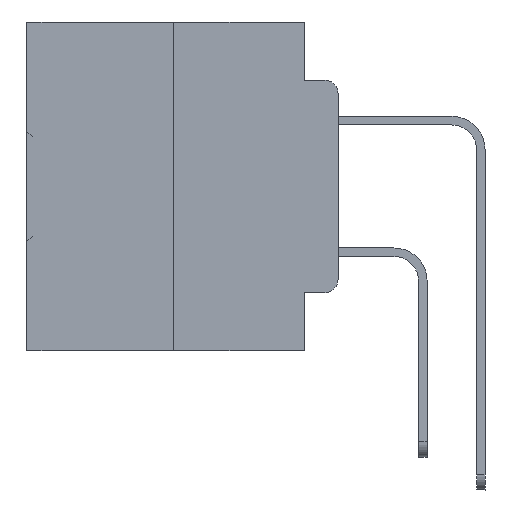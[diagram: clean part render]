
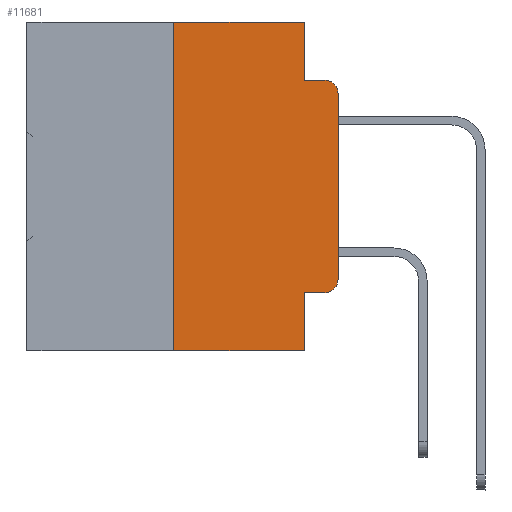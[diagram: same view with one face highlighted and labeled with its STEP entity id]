
A CAD part, left-side view. The second image highlights one B-rep face of the part: STEP entity #11681.
In plain terms, the highlighted planar face has unit normal (-1, 0, 0).
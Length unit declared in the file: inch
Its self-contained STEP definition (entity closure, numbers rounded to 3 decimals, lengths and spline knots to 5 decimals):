
#57 = AXIS2_PLACEMENT_3D ( 'NONE', #3207, #20721, #287 ) ;
#157 = EDGE_CURVE ( 'NONE', #1667, #24274, #2698, .T. ) ;
#287 = DIRECTION ( 'NONE',  ( 0., 0., -1. ) ) ;
#736 = AXIS2_PLACEMENT_3D ( 'NONE', #13805, #28581, #25678 ) ;
#817 = CARTESIAN_POINT ( 'NONE',  ( 0., 0.25, 0. ) ) ;
#1450 = ORIENTED_EDGE ( 'NONE', *, *, #25796, .F. ) ;
#1482 = DIRECTION ( 'NONE',  ( 0., -1., 0. ) ) ;
#1667 = VERTEX_POINT ( 'NONE', #22280 ) ;
#1740 = VECTOR ( 'NONE', #12706, 39.37008 ) ;
#2698 = LINE ( 'NONE', #18042, #23612 ) ;
#3207 = CARTESIAN_POINT ( 'NONE',  ( 0., 0.02, -0.1085 ) ) ;
#3311 = VERTEX_POINT ( 'NONE', #14318 ) ;
#4388 = VERTEX_POINT ( 'NONE', #18475 ) ;
#5861 = EDGE_LOOP ( 'NONE', ( #22556, #22879, #12348, #12440, #23515, #37566, #24303, #1450, #14983, #13837 ) ) ;
#7204 = LINE ( 'NONE', #817, #25745 ) ;
#7240 = FACE_OUTER_BOUND ( 'NONE', #5861, .T. ) ;
#7649 = DIRECTION ( 'NONE',  ( 0., 0., -1. ) ) ;
#7660 = EDGE_CURVE ( 'NONE', #4388, #3311, #16270, .T. ) ;
#8746 = CIRCLE ( 'NONE', #57, 0.02 ) ;
#9782 = EDGE_CURVE ( 'NONE', #13074, #14452, #31385, .T. ) ;
#9816 = DIRECTION ( 'NONE',  ( 0., 0., 1. ) ) ;
#10274 = EDGE_CURVE ( 'NONE', #3311, #13074, #19982, .T. ) ;
#11079 = VECTOR ( 'NONE', #33653, 39.37008 ) ;
#11506 = VERTEX_POINT ( 'NONE', #20715 ) ;
#11681 = ADVANCED_FACE ( 'NONE', ( #7240 ), #37041, .F. ) ;
#12348 = ORIENTED_EDGE ( 'NONE', *, *, #38094, .F. ) ;
#12440 = ORIENTED_EDGE ( 'NONE', *, *, #157, .F. ) ;
#12706 = DIRECTION ( 'NONE',  ( 0., -1., 0. ) ) ;
#13074 = VERTEX_POINT ( 'NONE', #14238 ) ;
#13103 = CARTESIAN_POINT ( 'NONE',  ( 0., 0.473, 0. ) ) ;
#13655 = DIRECTION ( 'NONE',  ( 1., 0., 0. ) ) ;
#13800 = VECTOR ( 'NONE', #36875, 39.37008 ) ;
#13805 = CARTESIAN_POINT ( 'NONE',  ( 0., 0.02, -0.3915 ) ) ;
#13837 = ORIENTED_EDGE ( 'NONE', *, *, #10274, .T. ) ;
#14238 = CARTESIAN_POINT ( 'NONE',  ( 0., 0., -0.3915 ) ) ;
#14318 = CARTESIAN_POINT ( 'NONE',  ( 0., 0.02, -0.4115 ) ) ;
#14452 = VERTEX_POINT ( 'NONE', #27267 ) ;
#14475 = VECTOR ( 'NONE', #36356, 39.37008 ) ;
#14983 = ORIENTED_EDGE ( 'NONE', *, *, #7660, .T. ) ;
#16270 = LINE ( 'NONE', #19168, #33511 ) ;
#16288 = CARTESIAN_POINT ( 'NONE',  ( 0., 0.051, -0.0885 ) ) ;
#18042 = CARTESIAN_POINT ( 'NONE',  ( 0., 0.051, 0. ) ) ;
#18265 = LINE ( 'NONE', #30523, #11079 ) ;
#18475 = CARTESIAN_POINT ( 'NONE',  ( 0., 0.051, -0.4115 ) ) ;
#19102 = CARTESIAN_POINT ( 'NONE',  ( 0., 0.473, 0. ) ) ;
#19168 = CARTESIAN_POINT ( 'NONE',  ( 0., 0.051, -0.4115 ) ) ;
#19514 = LINE ( 'NONE', #13103, #13800 ) ;
#19728 = VERTEX_POINT ( 'NONE', #36429 ) ;
#19982 = CIRCLE ( 'NONE', #736, 0.02 ) ;
#20651 = EDGE_CURVE ( 'NONE', #32588, #1667, #19514, .T. ) ;
#20715 = CARTESIAN_POINT ( 'NONE',  ( 0., 0.051, -0.5 ) ) ;
#20721 = DIRECTION ( 'NONE',  ( -1., 0., 0. ) ) ;
#21841 = AXIS2_PLACEMENT_3D ( 'NONE', #19102, #13655, #7649 ) ;
#22280 = CARTESIAN_POINT ( 'NONE',  ( 0., 0.051, 0. ) ) ;
#22556 = ORIENTED_EDGE ( 'NONE', *, *, #9782, .T. ) ;
#22779 = EDGE_CURVE ( 'NONE', #32315, #32588, #7204, .T. ) ;
#22879 = ORIENTED_EDGE ( 'NONE', *, *, #34409, .T. ) ;
#23515 = ORIENTED_EDGE ( 'NONE', *, *, #20651, .F. ) ;
#23612 = VECTOR ( 'NONE', #23697, 39.37008 ) ;
#23697 = DIRECTION ( 'NONE',  ( 0., 0., -1. ) ) ;
#24274 = VERTEX_POINT ( 'NONE', #16288 ) ;
#24303 = ORIENTED_EDGE ( 'NONE', *, *, #25212, .T. ) ;
#25151 = LINE ( 'NONE', #33365, #1740 ) ;
#25212 = EDGE_CURVE ( 'NONE', #32315, #11506, #25151, .T. ) ;
#25678 = DIRECTION ( 'NONE',  ( 0., 0., -1. ) ) ;
#25725 = CARTESIAN_POINT ( 'NONE',  ( 0., 0., 0. ) ) ;
#25745 = VECTOR ( 'NONE', #27660, 39.37008 ) ;
#25796 = EDGE_CURVE ( 'NONE', #4388, #11506, #18265, .T. ) ;
#27267 = CARTESIAN_POINT ( 'NONE',  ( 0., 0., -0.1085 ) ) ;
#27660 = DIRECTION ( 'NONE',  ( 0., 0., 1. ) ) ;
#27764 = LINE ( 'NONE', #35978, #14475 ) ;
#28581 = DIRECTION ( 'NONE',  ( -1., 0., 0. ) ) ;
#30523 = CARTESIAN_POINT ( 'NONE',  ( 0., 0.051, 0. ) ) ;
#31385 = LINE ( 'NONE', #25725, #33037 ) ;
#32315 = VERTEX_POINT ( 'NONE', #36543 ) ;
#32588 = VERTEX_POINT ( 'NONE', #37529 ) ;
#33037 = VECTOR ( 'NONE', #9816, 39.37008 ) ;
#33365 = CARTESIAN_POINT ( 'NONE',  ( 0., 0.473, -0.5 ) ) ;
#33511 = VECTOR ( 'NONE', #1482, 39.37008 ) ;
#33653 = DIRECTION ( 'NONE',  ( 0., 0., -1. ) ) ;
#34409 = EDGE_CURVE ( 'NONE', #14452, #19728, #8746, .T. ) ;
#35978 = CARTESIAN_POINT ( 'NONE',  ( 0., 0.051, -0.0885 ) ) ;
#36356 = DIRECTION ( 'NONE',  ( 0., -1., 0. ) ) ;
#36429 = CARTESIAN_POINT ( 'NONE',  ( 0., 0.02, -0.0885 ) ) ;
#36543 = CARTESIAN_POINT ( 'NONE',  ( 0., 0.25, -0.5 ) ) ;
#36875 = DIRECTION ( 'NONE',  ( 0., -1., 0. ) ) ;
#37041 = PLANE ( 'NONE',  #21841 ) ;
#37529 = CARTESIAN_POINT ( 'NONE',  ( 0., 0.25, 0. ) ) ;
#37566 = ORIENTED_EDGE ( 'NONE', *, *, #22779, .F. ) ;
#38094 = EDGE_CURVE ( 'NONE', #24274, #19728, #27764, .T. ) ;
